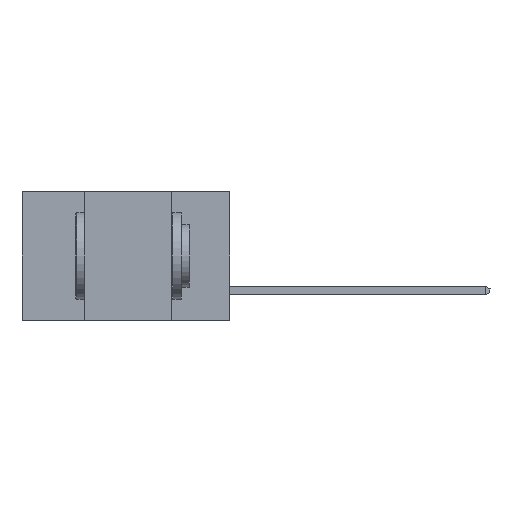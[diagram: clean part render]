
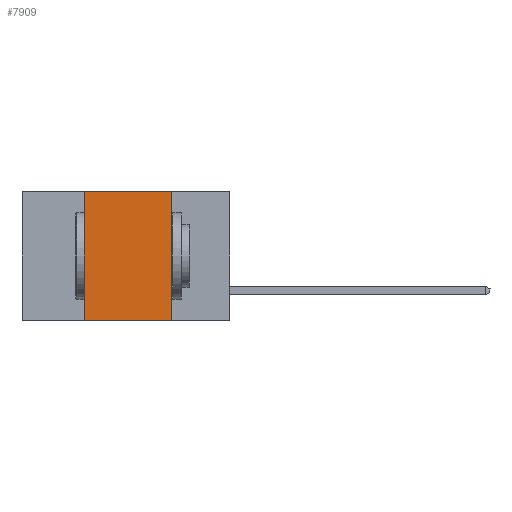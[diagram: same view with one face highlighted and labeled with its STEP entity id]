
A CAD part, left-side view. The second image highlights one B-rep face of the part: STEP entity #7909.
In plain terms, the highlighted planar face has unit normal (-1, 0, 0).
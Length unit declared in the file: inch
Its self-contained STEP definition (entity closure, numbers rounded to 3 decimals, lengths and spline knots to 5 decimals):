
#146 = ORIENTED_EDGE ( 'NONE', *, *, #11083, .F. ) ;
#769 = VECTOR ( 'NONE', #1003, 39.37008 ) ;
#808 = DIRECTION ( 'NONE',  ( 0., 0., -1. ) ) ;
#978 = VECTOR ( 'NONE', #10489, 39.37008 ) ;
#1003 = DIRECTION ( 'NONE',  ( 0., 0., 1. ) ) ;
#1242 = LINE ( 'NONE', #12929, #5450 ) ;
#1767 = EDGE_CURVE ( 'NONE', #6476, #11127, #14193, .T. ) ;
#1958 = AXIS2_PLACEMENT_3D ( 'NONE', #4622, #6843, #808 ) ;
#3076 = ORIENTED_EDGE ( 'NONE', *, *, #1767, .F. ) ;
#3116 = LINE ( 'NONE', #12608, #769 ) ;
#3725 = CARTESIAN_POINT ( 'NONE',  ( 0., 0.17, -0.37 ) ) ;
#4113 = CARTESIAN_POINT ( 'NONE',  ( 0., 0.42, 0. ) ) ;
#4475 = VERTEX_POINT ( 'NONE', #14670 ) ;
#4622 = CARTESIAN_POINT ( 'NONE',  ( 0., 0.6, 0. ) ) ;
#5421 = CARTESIAN_POINT ( 'NONE',  ( 0., 0.6, -0.37 ) ) ;
#5450 = VECTOR ( 'NONE', #10451, 39.37008 ) ;
#5637 = CARTESIAN_POINT ( 'NONE',  ( 0., 0.17, 0. ) ) ;
#6476 = VERTEX_POINT ( 'NONE', #5637 ) ;
#6623 = EDGE_CURVE ( 'NONE', #11400, #6476, #1242, .T. ) ;
#6843 = DIRECTION ( 'NONE',  ( 1., 0., 0. ) ) ;
#7700 = VECTOR ( 'NONE', #10097, 39.37008 ) ;
#7770 = EDGE_CURVE ( 'NONE', #4475, #11127, #12573, .T. ) ;
#7909 = ADVANCED_FACE ( 'NONE', ( #13954 ), #14105, .F. ) ;
#8321 = CARTESIAN_POINT ( 'NONE',  ( 0., 0.17, -0.37 ) ) ;
#9341 = ORIENTED_EDGE ( 'NONE', *, *, #7770, .T. ) ;
#10097 = DIRECTION ( 'NONE',  ( 0., -1., 0. ) ) ;
#10169 = EDGE_LOOP ( 'NONE', ( #3076, #11682, #146, #9341 ) ) ;
#10451 = DIRECTION ( 'NONE',  ( 0., -1., 0. ) ) ;
#10489 = DIRECTION ( 'NONE',  ( 0., 0., -1. ) ) ;
#11083 = EDGE_CURVE ( 'NONE', #4475, #11400, #3116, .T. ) ;
#11127 = VERTEX_POINT ( 'NONE', #3725 ) ;
#11400 = VERTEX_POINT ( 'NONE', #4113 ) ;
#11682 = ORIENTED_EDGE ( 'NONE', *, *, #6623, .F. ) ;
#12573 = LINE ( 'NONE', #5421, #7700 ) ;
#12608 = CARTESIAN_POINT ( 'NONE',  ( 0., 0.42, -0.37 ) ) ;
#12929 = CARTESIAN_POINT ( 'NONE',  ( 0., 0.6, 0. ) ) ;
#13954 = FACE_OUTER_BOUND ( 'NONE', #10169, .T. ) ;
#14105 = PLANE ( 'NONE',  #1958 ) ;
#14193 = LINE ( 'NONE', #8321, #978 ) ;
#14670 = CARTESIAN_POINT ( 'NONE',  ( 0., 0.42, -0.37 ) ) ;
